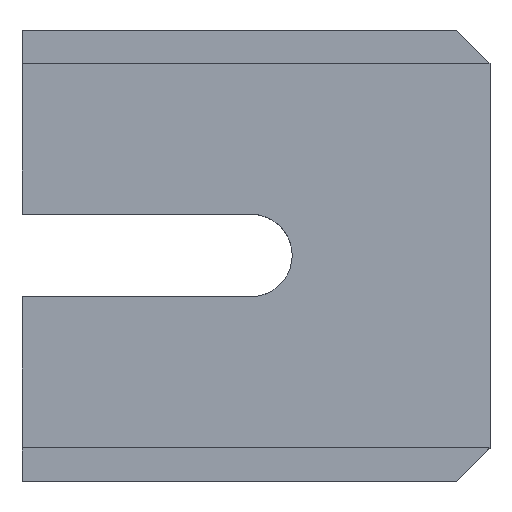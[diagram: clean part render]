
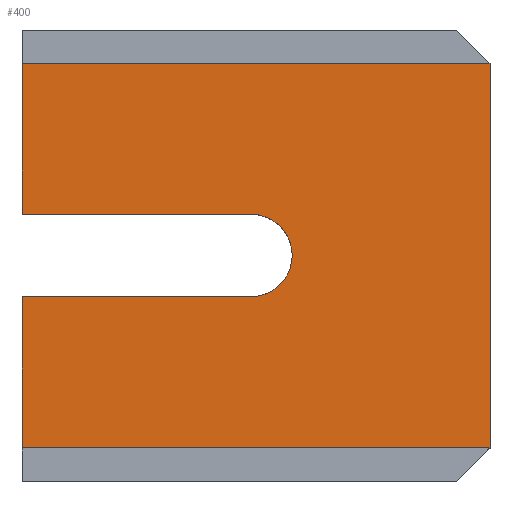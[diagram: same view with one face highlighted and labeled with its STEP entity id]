
A CAD part, top view. The second image highlights one B-rep face of the part: STEP entity #400.
In plain terms, the highlighted planar face has unit normal (0, 0, 1).
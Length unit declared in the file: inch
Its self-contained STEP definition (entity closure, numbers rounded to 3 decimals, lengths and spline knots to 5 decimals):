
#23=CIRCLE('',#439,0.08268);
#41=FACE_OUTER_BOUND('',#63,.T.);
#63=EDGE_LOOP('',(#325,#326,#327,#328,#329,#330,#331,#332));
#79=LINE('',#578,#127);
#92=LINE('',#608,#140);
#97=LINE('',#620,#145);
#102=LINE('',#629,#150);
#105=LINE('',#658,#153);
#112=LINE('',#673,#160);
#113=LINE('',#674,#161);
#127=VECTOR('',#470,0.3937);
#140=VECTOR('',#493,0.3937);
#145=VECTOR('',#502,0.3937);
#150=VECTOR('',#509,0.3937);
#153=VECTOR('',#522,0.3937);
#160=VECTOR('',#537,0.3937);
#161=VECTOR('',#538,0.3937);
#173=VERTEX_POINT('',#575);
#174=VERTEX_POINT('',#577);
#185=VERTEX_POINT('',#606);
#186=VERTEX_POINT('',#607);
#191=VERTEX_POINT('',#618);
#194=VERTEX_POINT('',#627);
#196=VERTEX_POINT('',#655);
#201=VERTEX_POINT('',#672);
#211=EDGE_CURVE('',#173,#174,#79,.T.);
#225=EDGE_CURVE('',#185,#186,#92,.T.);
#231=EDGE_CURVE('',#191,#173,#97,.T.);
#236=EDGE_CURVE('',#191,#194,#102,.T.);
#237=EDGE_CURVE('',#194,#185,#23,.T.);
#242=EDGE_CURVE('',#196,#186,#105,.T.);
#250=EDGE_CURVE('',#201,#196,#112,.T.);
#251=EDGE_CURVE('',#201,#174,#113,.T.);
#325=ORIENTED_EDGE('',*,*,#225,.T.);
#326=ORIENTED_EDGE('',*,*,#242,.F.);
#327=ORIENTED_EDGE('',*,*,#250,.F.);
#328=ORIENTED_EDGE('',*,*,#251,.T.);
#329=ORIENTED_EDGE('',*,*,#211,.F.);
#330=ORIENTED_EDGE('',*,*,#231,.F.);
#331=ORIENTED_EDGE('',*,*,#236,.T.);
#332=ORIENTED_EDGE('',*,*,#237,.T.);
#380=PLANE('',#446);
#400=ADVANCED_FACE('',(#41),#380,.T.);
#439=AXIS2_PLACEMENT_3D('',#631,#512,#513);
#446=AXIS2_PLACEMENT_3D('',#671,#535,#536);
#470=DIRECTION('',(1.,0.,0.));
#493=DIRECTION('',(-1.,0.,0.));
#502=DIRECTION('',(0.,1.,0.));
#509=DIRECTION('',(1.,0.,0.));
#512=DIRECTION('center_axis',(0.,0.,-1.));
#513=DIRECTION('ref_axis',(1.,0.,0.));
#522=DIRECTION('',(0.,1.,0.));
#535=DIRECTION('center_axis',(0.,0.,1.));
#536=DIRECTION('ref_axis',(1.,0.,0.));
#537=DIRECTION('',(-1.,0.,0.));
#538=DIRECTION('',(0.,1.,0.));
#575=CARTESIAN_POINT('',(0.7874,0.38527,-1.02567));
#577=CARTESIAN_POINT('',(1.72657,0.38527,-1.02567));
#578=CARTESIAN_POINT('',(1.72657,0.38527,-1.02567));
#606=CARTESIAN_POINT('',(1.24701,-0.08268,-1.02567));
#607=CARTESIAN_POINT('',(0.7874,-0.08268,-1.02567));
#608=CARTESIAN_POINT('',(1.01228,-0.08268,-1.02567));
#618=CARTESIAN_POINT('',(0.7874,0.08268,-1.02567));
#620=CARTESIAN_POINT('',(0.7874,0.,-1.02567));
#627=CARTESIAN_POINT('',(1.24701,0.08268,-1.02567));
#629=CARTESIAN_POINT('',(1.01228,0.08268,-1.02567));
#631=CARTESIAN_POINT('Origin',(1.24701,0.,-1.02567));
#655=CARTESIAN_POINT('',(0.7874,-0.38527,-1.02567));
#658=CARTESIAN_POINT('',(0.7874,0.,-1.02567));
#671=CARTESIAN_POINT('Origin',(0.7874,0.,-1.02567));
#672=CARTESIAN_POINT('',(1.72657,-0.38527,-1.02567));
#673=CARTESIAN_POINT('',(1.72657,-0.38527,-1.02567));
#674=CARTESIAN_POINT('',(1.72657,0.,-1.02567));
